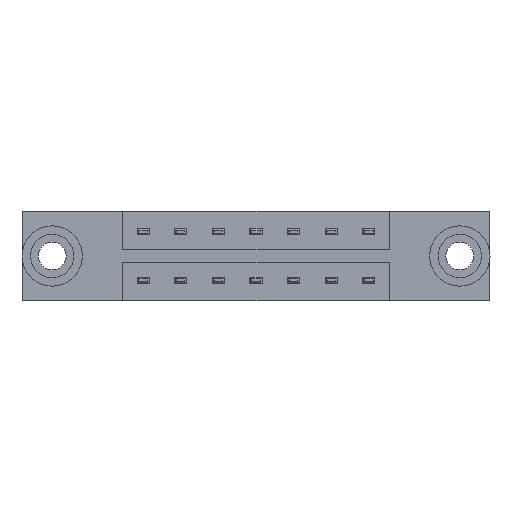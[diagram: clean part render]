
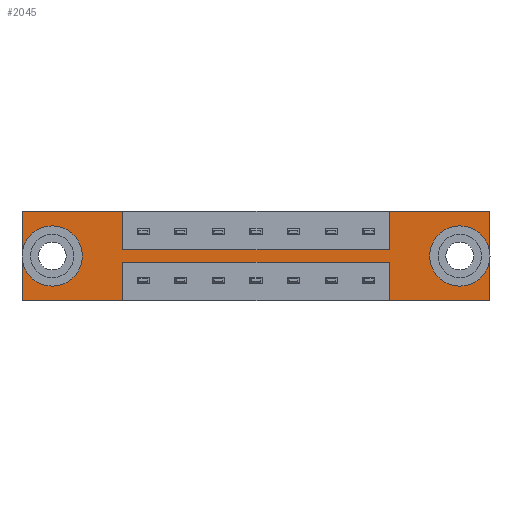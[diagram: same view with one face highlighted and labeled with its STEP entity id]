
A CAD part, front view. The second image highlights one B-rep face of the part: STEP entity #2045.
In plain terms, the highlighted planar face has unit normal (0, -1, 0).
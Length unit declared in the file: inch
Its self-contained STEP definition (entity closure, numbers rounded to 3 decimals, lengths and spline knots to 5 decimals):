
#63 = CARTESIAN_POINT ( 'NONE',  ( 1.5225, 0., -0.37 ) ) ;
#99 = EDGE_CURVE ( 'NONE', #8122, #1195, #7246, .T. ) ;
#228 = LINE ( 'NONE', #5515, #6701 ) ;
#326 = AXIS2_PLACEMENT_3D ( 'NONE', #9422, #8708, #2128 ) ;
#455 = CARTESIAN_POINT ( 'NONE',  ( 0., 0., 0. ) ) ;
#615 = EDGE_CURVE ( 'NONE', #3653, #2355, #5322, .T. ) ;
#648 = VERTEX_POINT ( 'NONE', #9059 ) ;
#687 = ORIENTED_EDGE ( 'NONE', *, *, #3673, .F. ) ;
#717 = EDGE_LOOP ( 'NONE', ( #8682, #5986 ) ) ;
#719 = FACE_BOUND ( 'NONE', #717, .T. ) ;
#807 = PLANE ( 'NONE',  #7896 ) ;
#893 = DIRECTION ( 'NONE',  ( 0., 1., 0. ) ) ;
#961 = CARTESIAN_POINT ( 'NONE',  ( 1.5225, 0., -0.1585 ) ) ;
#981 = DIRECTION ( 'NONE',  ( 0., 1., 0. ) ) ;
#1110 = DIRECTION ( 'NONE',  ( 0., 0., 1. ) ) ;
#1195 = VERTEX_POINT ( 'NONE', #3715 ) ;
#1273 = DIRECTION ( 'NONE',  ( 0., 0., 1. ) ) ;
#1315 = CARTESIAN_POINT ( 'NONE',  ( 1.94, 0., -0.37 ) ) ;
#1467 = CARTESIAN_POINT ( 'NONE',  ( 1.5225, 0., -0.1585 ) ) ;
#1496 = VECTOR ( 'NONE', #3401, 39.37008 ) ;
#1522 = DIRECTION ( 'NONE',  ( -1., 0., 0. ) ) ;
#1523 = LINE ( 'NONE', #4518, #4320 ) ;
#1825 = VERTEX_POINT ( 'NONE', #961 ) ;
#1835 = DIRECTION ( 'NONE',  ( 0., 0., 1. ) ) ;
#1899 = VECTOR ( 'NONE', #7648, 39.37008 ) ;
#2019 = EDGE_CURVE ( 'NONE', #1195, #7400, #7078, .T. ) ;
#2045 = ADVANCED_FACE ( 'NONE', ( #8928, #719, #6629 ), #807, .T. ) ;
#2062 = VECTOR ( 'NONE', #1522, 39.37008 ) ;
#2070 = CARTESIAN_POINT ( 'NONE',  ( 1.815, 0., -0.107 ) ) ;
#2128 = DIRECTION ( 'NONE',  ( 0., 0., 1. ) ) ;
#2194 = DIRECTION ( 'NONE',  ( 1., 0., 0. ) ) ;
#2251 = EDGE_CURVE ( 'NONE', #2283, #648, #3358, .T. ) ;
#2266 = CARTESIAN_POINT ( 'NONE',  ( 0.125, 0., -0.263 ) ) ;
#2283 = VERTEX_POINT ( 'NONE', #7740 ) ;
#2355 = VERTEX_POINT ( 'NONE', #2070 ) ;
#2407 = ORIENTED_EDGE ( 'NONE', *, *, #9195, .F. ) ;
#2409 = ORIENTED_EDGE ( 'NONE', *, *, #2251, .F. ) ;
#2802 = VERTEX_POINT ( 'NONE', #1315 ) ;
#2921 = CARTESIAN_POINT ( 'NONE',  ( 0.4175, 0., -0.1585 ) ) ;
#2971 = AXIS2_PLACEMENT_3D ( 'NONE', #5483, #981, #8290 ) ;
#3068 = ORIENTED_EDGE ( 'NONE', *, *, #8097, .F. ) ;
#3079 = CARTESIAN_POINT ( 'NONE',  ( 1.5225, 0., -0.2115 ) ) ;
#3095 = ORIENTED_EDGE ( 'NONE', *, *, #7416, .F. ) ;
#3100 = CARTESIAN_POINT ( 'NONE',  ( 1.815, 0., -0.185 ) ) ;
#3125 = ORIENTED_EDGE ( 'NONE', *, *, #99, .F. ) ;
#3270 = LINE ( 'NONE', #7558, #4377 ) ;
#3279 = DIRECTION ( 'NONE',  ( 0., 1., 0. ) ) ;
#3358 = LINE ( 'NONE', #6823, #1899 ) ;
#3373 = EDGE_CURVE ( 'NONE', #6335, #5992, #7576, .T. ) ;
#3401 = DIRECTION ( 'NONE',  ( 1., 0., 0. ) ) ;
#3418 = CIRCLE ( 'NONE', #2971, 0.078 ) ;
#3653 = VERTEX_POINT ( 'NONE', #4191 ) ;
#3661 = DIRECTION ( 'NONE',  ( 0., -1., 0. ) ) ;
#3673 = EDGE_CURVE ( 'NONE', #6663, #1825, #8779, .T. ) ;
#3712 = CARTESIAN_POINT ( 'NONE',  ( 0., 0., -0.37 ) ) ;
#3715 = CARTESIAN_POINT ( 'NONE',  ( 0.4175, 0., -0.37 ) ) ;
#3740 = DIRECTION ( 'NONE',  ( 0., 0., -1. ) ) ;
#3782 = EDGE_CURVE ( 'NONE', #2802, #6142, #5146, .T. ) ;
#3815 = DIRECTION ( 'NONE',  ( 0., 0., -1. ) ) ;
#3995 = EDGE_CURVE ( 'NONE', #5992, #6335, #4797, .T. ) ;
#4005 = CARTESIAN_POINT ( 'NONE',  ( 0.125, 0., -0.107 ) ) ;
#4075 = VECTOR ( 'NONE', #1273, 39.37008 ) ;
#4191 = CARTESIAN_POINT ( 'NONE',  ( 1.815, 0., -0.263 ) ) ;
#4272 = CARTESIAN_POINT ( 'NONE',  ( 0., 0., 0. ) ) ;
#4320 = VECTOR ( 'NONE', #8870, 39.37008 ) ;
#4377 = VECTOR ( 'NONE', #1835, 39.37008 ) ;
#4387 = CARTESIAN_POINT ( 'NONE',  ( 0.4175, 0., -0.2115 ) ) ;
#4440 = VERTEX_POINT ( 'NONE', #3079 ) ;
#4518 = CARTESIAN_POINT ( 'NONE',  ( 0.4175, 0., -0.2115 ) ) ;
#4583 = VERTEX_POINT ( 'NONE', #9129 ) ;
#4615 = EDGE_LOOP ( 'NONE', ( #6658, #6631 ) ) ;
#4719 = CARTESIAN_POINT ( 'NONE',  ( 0.4175, 0., -0.1585 ) ) ;
#4797 = CIRCLE ( 'NONE', #5236, 0.078 ) ;
#4799 = DIRECTION ( 'NONE',  ( 0., 0., 1. ) ) ;
#4894 = DIRECTION ( 'NONE',  ( -1., 0., 0. ) ) ;
#4949 = VECTOR ( 'NONE', #4894, 39.37008 ) ;
#4969 = ORIENTED_EDGE ( 'NONE', *, *, #2019, .F. ) ;
#5061 = ORIENTED_EDGE ( 'NONE', *, *, #7222, .F. ) ;
#5126 = CARTESIAN_POINT ( 'NONE',  ( 0., 0., -0.37 ) ) ;
#5135 = DIRECTION ( 'NONE',  ( 0., 0., -1. ) ) ;
#5146 = LINE ( 'NONE', #3712, #2062 ) ;
#5176 = CARTESIAN_POINT ( 'NONE',  ( 1.94, 0., 0. ) ) ;
#5236 = AXIS2_PLACEMENT_3D ( 'NONE', #6258, #3279, #1110 ) ;
#5322 = CIRCLE ( 'NONE', #9023, 0.078 ) ;
#5410 = ORIENTED_EDGE ( 'NONE', *, *, #8725, .F. ) ;
#5480 = EDGE_CURVE ( 'NONE', #4583, #6663, #7854, .T. ) ;
#5483 = CARTESIAN_POINT ( 'NONE',  ( 1.815, 0., -0.185 ) ) ;
#5515 = CARTESIAN_POINT ( 'NONE',  ( 0., 0., 0. ) ) ;
#5961 = EDGE_LOOP ( 'NONE', ( #5410, #7991, #5061, #2409, #2407, #687, #6359, #3095, #6506, #4969, #3125, #3068 ) ) ;
#5965 = CARTESIAN_POINT ( 'NONE',  ( 0.4175, 0., -0.2115 ) ) ;
#5986 = ORIENTED_EDGE ( 'NONE', *, *, #3995, .T. ) ;
#5992 = VERTEX_POINT ( 'NONE', #2266 ) ;
#6142 = VERTEX_POINT ( 'NONE', #63 ) ;
#6258 = CARTESIAN_POINT ( 'NONE',  ( 0.125, 0., -0.185 ) ) ;
#6335 = VERTEX_POINT ( 'NONE', #4005 ) ;
#6336 = VECTOR ( 'NONE', #2194, 39.37008 ) ;
#6356 = LINE ( 'NONE', #1467, #4075 ) ;
#6359 = ORIENTED_EDGE ( 'NONE', *, *, #5480, .F. ) ;
#6506 = ORIENTED_EDGE ( 'NONE', *, *, #9484, .F. ) ;
#6545 = VECTOR ( 'NONE', #5135, 39.37008 ) ;
#6629 = FACE_OUTER_BOUND ( 'NONE', #5961, .T. ) ;
#6631 = ORIENTED_EDGE ( 'NONE', *, *, #615, .T. ) ;
#6658 = ORIENTED_EDGE ( 'NONE', *, *, #7861, .T. ) ;
#6663 = VERTEX_POINT ( 'NONE', #4719 ) ;
#6701 = VECTOR ( 'NONE', #4799, 39.37008 ) ;
#6823 = CARTESIAN_POINT ( 'NONE',  ( 0., 0., 0. ) ) ;
#7078 = LINE ( 'NONE', #9283, #4949 ) ;
#7114 = VERTEX_POINT ( 'NONE', #4272 ) ;
#7128 = CARTESIAN_POINT ( 'NONE',  ( 0.4175, 0., -0.1585 ) ) ;
#7222 = EDGE_CURVE ( 'NONE', #648, #2802, #8859, .T. ) ;
#7246 = LINE ( 'NONE', #4387, #7994 ) ;
#7400 = VERTEX_POINT ( 'NONE', #8497 ) ;
#7416 = EDGE_CURVE ( 'NONE', #7114, #4583, #7788, .T. ) ;
#7558 = CARTESIAN_POINT ( 'NONE',  ( 1.5225, 0., -0.2115 ) ) ;
#7576 = CIRCLE ( 'NONE', #326, 0.078 ) ;
#7648 = DIRECTION ( 'NONE',  ( 1., 0., 0. ) ) ;
#7740 = CARTESIAN_POINT ( 'NONE',  ( 1.5225, 0., 0. ) ) ;
#7788 = LINE ( 'NONE', #455, #1496 ) ;
#7854 = LINE ( 'NONE', #7128, #8208 ) ;
#7861 = EDGE_CURVE ( 'NONE', #2355, #3653, #3418, .T. ) ;
#7896 = AXIS2_PLACEMENT_3D ( 'NONE', #5126, #3661, #3740 ) ;
#7973 = DIRECTION ( 'NONE',  ( 0., 0., -1. ) ) ;
#7991 = ORIENTED_EDGE ( 'NONE', *, *, #3782, .F. ) ;
#7994 = VECTOR ( 'NONE', #7973, 39.37008 ) ;
#8097 = EDGE_CURVE ( 'NONE', #4440, #8122, #1523, .T. ) ;
#8122 = VERTEX_POINT ( 'NONE', #5965 ) ;
#8208 = VECTOR ( 'NONE', #9231, 39.37008 ) ;
#8290 = DIRECTION ( 'NONE',  ( 0., 0., -1. ) ) ;
#8497 = CARTESIAN_POINT ( 'NONE',  ( 0., 0., -0.37 ) ) ;
#8682 = ORIENTED_EDGE ( 'NONE', *, *, #3373, .T. ) ;
#8708 = DIRECTION ( 'NONE',  ( 0., 1., 0. ) ) ;
#8725 = EDGE_CURVE ( 'NONE', #6142, #4440, #3270, .T. ) ;
#8779 = LINE ( 'NONE', #2921, #6336 ) ;
#8859 = LINE ( 'NONE', #5176, #6545 ) ;
#8870 = DIRECTION ( 'NONE',  ( -1., 0., 0. ) ) ;
#8928 = FACE_BOUND ( 'NONE', #4615, .T. ) ;
#9023 = AXIS2_PLACEMENT_3D ( 'NONE', #3100, #893, #3815 ) ;
#9059 = CARTESIAN_POINT ( 'NONE',  ( 1.94, 0., 0. ) ) ;
#9129 = CARTESIAN_POINT ( 'NONE',  ( 0.4175, 0., 0. ) ) ;
#9195 = EDGE_CURVE ( 'NONE', #1825, #2283, #6356, .T. ) ;
#9231 = DIRECTION ( 'NONE',  ( 0., 0., -1. ) ) ;
#9283 = CARTESIAN_POINT ( 'NONE',  ( 0., 0., -0.37 ) ) ;
#9422 = CARTESIAN_POINT ( 'NONE',  ( 0.125, 0., -0.185 ) ) ;
#9484 = EDGE_CURVE ( 'NONE', #7400, #7114, #228, .T. ) ;
